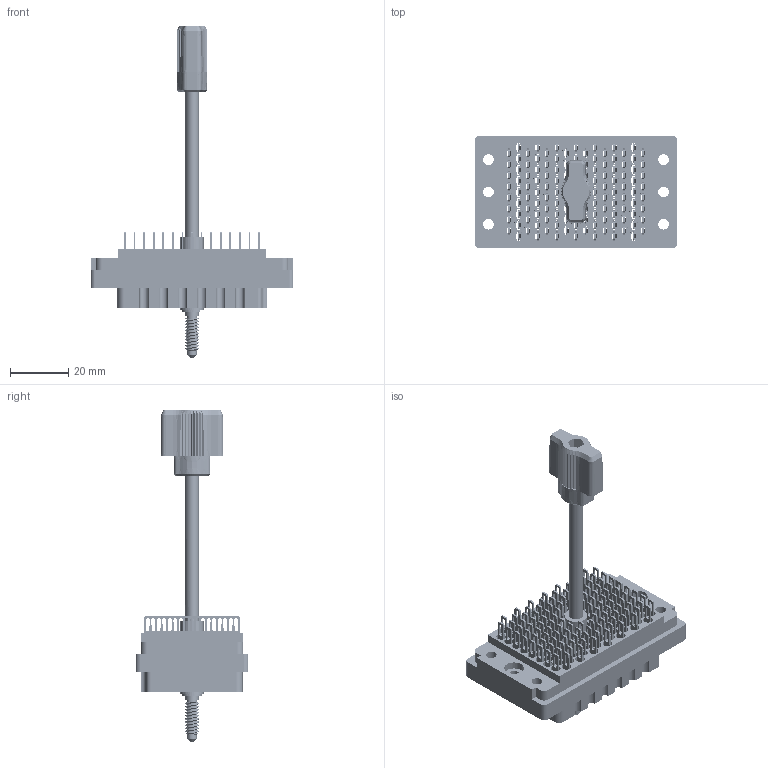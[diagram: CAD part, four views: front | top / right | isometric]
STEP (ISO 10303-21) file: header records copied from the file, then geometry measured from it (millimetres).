
FILE_DESCRIPTION (( 'STEP AP203' ), '1' );
FILE_NAME ('516-120-500-405.STEP', '2020-03-07T00:44:07', ( '' ), ( '' ), 'SwSTEP 2.0', 'SolidWorks 2016', '' );
FILE_SCHEMA (( 'CONFIG_CONTROL_DESIGN' ));
Length unit declared in the file: inch
Products named in the file (10): 516-251-095-100; 516-254-091-109; Grub Screw; 516-253-190-107; Actuating Screw Assy 090-120; 516-253-095-100; 516-120-500-405; 516-292-001_500 Contact; 516-250-091-111; 516 Part Receptacle_120
Assembly tree (129 placements, depth 3):
  516-120-500-405
    516 Part Receptacle_120
    516-292-001_500 Contact  x120
    Actuating Screw Assy 090-120
      516-251-095-100
      516-254-091-109
      516-253-095-100  x2
      516-253-190-107
      516-250-091-111
      Grub Screw
Bounding box: 69.85 x 38.73 x 114.34 mm (x, y, z)
Volume: 33976 mm3; surface area: 63783.4 mm2
Topology: 128 solids, 128 shells, 11909 faces, 34563 edges, 22934 vertices
Faces by surface type: plane 7063, cylinder 4047, bspline 737, cone 62
Entity records: 107176 total; most frequent: CARTESIAN_POINT 24488, ORIENTED_EDGE 16742, DIRECTION 16213, EDGE_CURVE 8371, LINE 6005, VECTOR 6005, VERTEX_POINT 5552, AXIS2_PLACEMENT_3D 5104
